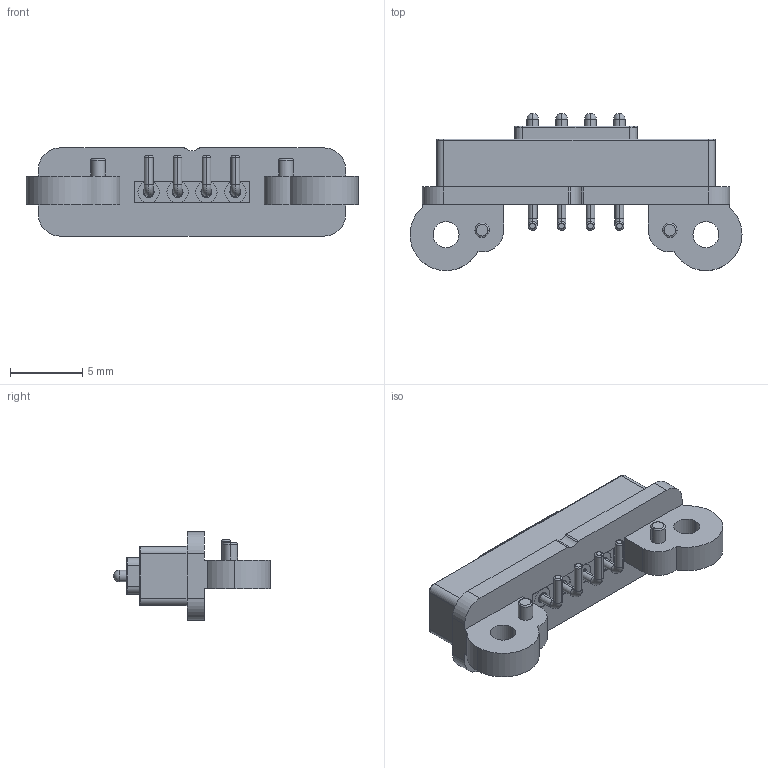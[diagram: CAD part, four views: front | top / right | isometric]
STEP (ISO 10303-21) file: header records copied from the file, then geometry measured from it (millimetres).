
FILE_DESCRIPTION (( 'STEP AP214' ), '1' );
FILE_NAME ('685J0421351124E.STEP', '2023-05-01T19:01:07', ( '' ), ( '' ), 'SwSTEP 2.0', 'SolidWorks 2020', '' );
FILE_SCHEMA (( 'AUTOMOTIVE_DESIGN' ));
Length unit declared in the file: inch
Products named in the file (1): 685J0421351124E
Bounding box: 23 x 10.89 x 6.1 mm (x, y, z)
Volume: 524.4 mm3; surface area: 683.8 mm2
Topology: 9 solids, 9 shells, 219 faces, 510 edges, 320 vertices
Faces by surface type: cylinder 92, plane 70, torus 36, bspline 13, sphere 8
Entity records: 9857 total; most frequent: CARTESIAN_POINT 1831, DIRECTION 1130, ORIENTED_EDGE 988, EDGE_CURVE 494, AXIS2_PLACEMENT_3D 455, VERTEX_POINT 312, CIRCLE 248, EDGE_LOOP 242
